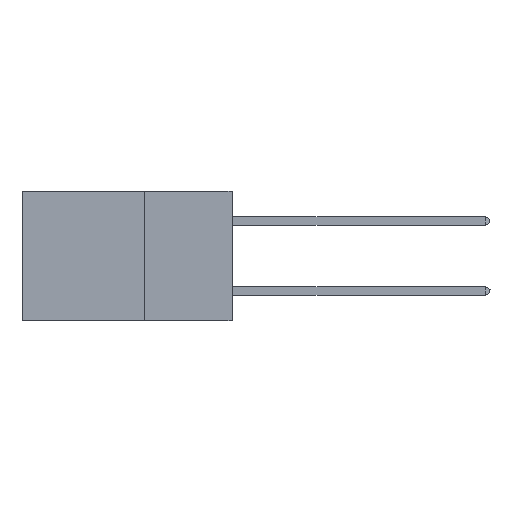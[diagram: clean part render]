
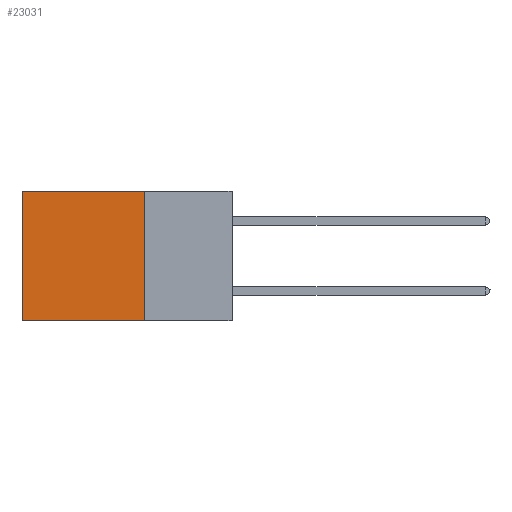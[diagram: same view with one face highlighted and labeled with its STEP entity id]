
A CAD part, left-side view. The second image highlights one B-rep face of the part: STEP entity #23031.
In plain terms, the highlighted planar face has unit normal (-1, 0, 0).
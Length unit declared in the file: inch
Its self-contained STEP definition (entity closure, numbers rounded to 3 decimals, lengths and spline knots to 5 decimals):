
#401 = DIRECTION ( 'NONE',  ( 1., 0., 0. ) ) ;
#1466 = EDGE_CURVE ( 'NONE', #31383, #2420, #25953, .T. ) ;
#2420 = VERTEX_POINT ( 'NONE', #28618 ) ;
#3845 = CARTESIAN_POINT ( 'NONE',  ( 0.2875, 0.25, -0.37 ) ) ;
#4533 = CARTESIAN_POINT ( 'NONE',  ( 0.2875, 0.25, 0. ) ) ;
#5267 = VECTOR ( 'NONE', #29983, 39.37008 ) ;
#6451 = CARTESIAN_POINT ( 'NONE',  ( 0.2875, 0.25, 0. ) ) ;
#7313 = CARTESIAN_POINT ( 'NONE',  ( 0.2875, 0.25, -0.37 ) ) ;
#8026 = EDGE_CURVE ( 'NONE', #22237, #31383, #17542, .T. ) ;
#8645 = ORIENTED_EDGE ( 'NONE', *, *, #8026, .F. ) ;
#8835 = VECTOR ( 'NONE', #10106, 39.37008 ) ;
#10106 = DIRECTION ( 'NONE',  ( 0., 1., 0. ) ) ;
#10829 = LINE ( 'NONE', #6451, #15518 ) ;
#11260 = EDGE_CURVE ( 'NONE', #25497, #2420, #16529, .T. ) ;
#13681 = VECTOR ( 'NONE', #22285, 39.37008 ) ;
#14707 = AXIS2_PLACEMENT_3D ( 'NONE', #14936, #401, #21322 ) ;
#14936 = CARTESIAN_POINT ( 'NONE',  ( 0.2875, 0.25, 0. ) ) ;
#15518 = VECTOR ( 'NONE', #33812, 39.37008 ) ;
#16529 = LINE ( 'NONE', #19070, #5267 ) ;
#17542 = LINE ( 'NONE', #30889, #13681 ) ;
#19070 = CARTESIAN_POINT ( 'NONE',  ( 0.2875, 0.6, 0. ) ) ;
#19117 = FACE_OUTER_BOUND ( 'NONE', #29128, .T. ) ;
#19853 = ORIENTED_EDGE ( 'NONE', *, *, #1466, .F. ) ;
#21322 = DIRECTION ( 'NONE',  ( 0., 0., -1. ) ) ;
#21429 = CARTESIAN_POINT ( 'NONE',  ( 0.2875, 0.6, 0. ) ) ;
#21715 = ORIENTED_EDGE ( 'NONE', *, *, #11260, .T. ) ;
#22237 = VERTEX_POINT ( 'NONE', #4533 ) ;
#22285 = DIRECTION ( 'NONE',  ( 0., 0., -1. ) ) ;
#23031 = ADVANCED_FACE ( 'NONE', ( #19117 ), #29079, .F. ) ;
#25497 = VERTEX_POINT ( 'NONE', #21429 ) ;
#25953 = LINE ( 'NONE', #7313, #8835 ) ;
#27877 = EDGE_CURVE ( 'NONE', #22237, #25497, #10829, .T. ) ;
#28618 = CARTESIAN_POINT ( 'NONE',  ( 0.2875, 0.6, -0.37 ) ) ;
#29079 = PLANE ( 'NONE',  #14707 ) ;
#29128 = EDGE_LOOP ( 'NONE', ( #21715, #19853, #8645, #33585 ) ) ;
#29983 = DIRECTION ( 'NONE',  ( 0., 0., -1. ) ) ;
#30889 = CARTESIAN_POINT ( 'NONE',  ( 0.2875, 0.25, 0. ) ) ;
#31383 = VERTEX_POINT ( 'NONE', #3845 ) ;
#33585 = ORIENTED_EDGE ( 'NONE', *, *, #27877, .T. ) ;
#33812 = DIRECTION ( 'NONE',  ( 0., 1., 0. ) ) ;
